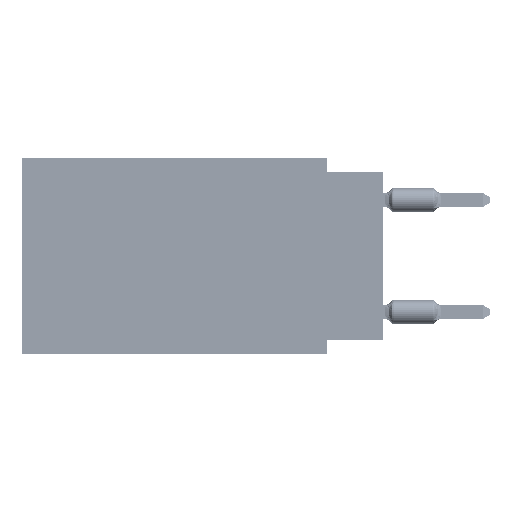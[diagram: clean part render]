
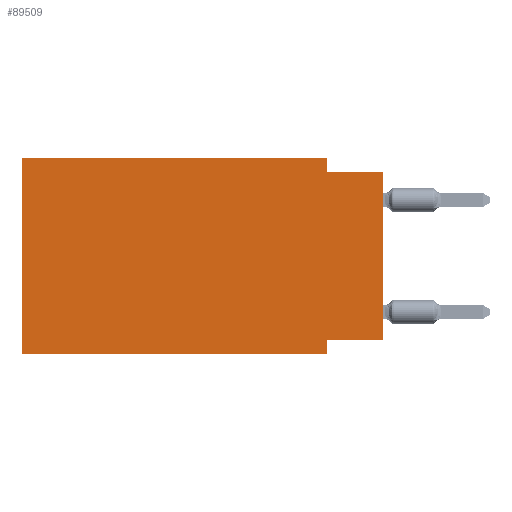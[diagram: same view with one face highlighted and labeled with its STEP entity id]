
A CAD part, left-side view. The second image highlights one B-rep face of the part: STEP entity #89509.
In plain terms, the highlighted planar face has unit normal (-1, 0, 0).
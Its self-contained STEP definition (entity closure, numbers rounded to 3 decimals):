
#2604 = DIRECTION ( 'NONE',  ( 0., 0., -1. ) ) ;
#7927 = EDGE_CURVE ( 'NONE', #21733, #20440, #15681, .T. ) ;
#8365 = CARTESIAN_POINT ( 'NONE',  ( 0., 16.383, -8.89 ) ) ;
#8653 = VECTOR ( 'NONE', #2604, 1000. ) ;
#8928 = DIRECTION ( 'NONE',  ( 0., -1., 0. ) ) ;
#9416 = CARTESIAN_POINT ( 'NONE',  ( 0., 16.383, 0. ) ) ;
#9968 = DIRECTION ( 'NONE',  ( 0., 0., -1. ) ) ;
#9999 = VECTOR ( 'NONE', #70797, 1000. ) ;
#10067 = DIRECTION ( 'NONE',  ( 0., 0., 1. ) ) ;
#15681 = LINE ( 'NONE', #32396, #109219 ) ;
#18236 = ORIENTED_EDGE ( 'NONE', *, *, #20844, .F. ) ;
#20440 = VERTEX_POINT ( 'NONE', #44941 ) ;
#20844 = EDGE_CURVE ( 'NONE', #87020, #33967, #105985, .T. ) ;
#21031 = CARTESIAN_POINT ( 'NONE',  ( 0., 2.54, 0. ) ) ;
#21733 = VERTEX_POINT ( 'NONE', #104017 ) ;
#23191 = CARTESIAN_POINT ( 'NONE',  ( 0., 2.54, -8.89 ) ) ;
#24398 = EDGE_CURVE ( 'NONE', #94822, #26685, #70625, .T. ) ;
#25597 = ORIENTED_EDGE ( 'NONE', *, *, #54971, .F. ) ;
#26632 = VECTOR ( 'NONE', #39932, 1000. ) ;
#26685 = VERTEX_POINT ( 'NONE', #106906 ) ;
#27922 = CARTESIAN_POINT ( 'NONE',  ( 0., 0., 0. ) ) ;
#28302 = VERTEX_POINT ( 'NONE', #31006 ) ;
#30061 = CARTESIAN_POINT ( 'NONE',  ( 0., 16.383, 0. ) ) ;
#30496 = VERTEX_POINT ( 'NONE', #94776 ) ;
#31006 = CARTESIAN_POINT ( 'NONE',  ( 0., 2.54, -0.635 ) ) ;
#32396 = CARTESIAN_POINT ( 'NONE',  ( 0., 16.383, 0. ) ) ;
#33326 = VECTOR ( 'NONE', #39279, 1000. ) ;
#33967 = VERTEX_POINT ( 'NONE', #63961 ) ;
#35767 = DIRECTION ( 'NONE',  ( 0., -1., 0. ) ) ;
#38302 = ORIENTED_EDGE ( 'NONE', *, *, #90954, .T. ) ;
#39279 = DIRECTION ( 'NONE',  ( 0., 0., 1. ) ) ;
#39932 = DIRECTION ( 'NONE',  ( 0., 0., -1. ) ) ;
#40236 = EDGE_CURVE ( 'NONE', #33967, #26685, #84927, .T. ) ;
#44941 = CARTESIAN_POINT ( 'NONE',  ( 0., 2.54, 0. ) ) ;
#46829 = FACE_OUTER_BOUND ( 'NONE', #102808, .T. ) ;
#54971 = EDGE_CURVE ( 'NONE', #20440, #28302, #64884, .T. ) ;
#60241 = ORIENTED_EDGE ( 'NONE', *, *, #78109, .F. ) ;
#63961 = CARTESIAN_POINT ( 'NONE',  ( 0., 2.54, -8.255 ) ) ;
#64884 = LINE ( 'NONE', #21031, #8653 ) ;
#66978 = LINE ( 'NONE', #30061, #33326 ) ;
#67086 = CARTESIAN_POINT ( 'NONE',  ( 0., 16.383, -8.89 ) ) ;
#70423 = LINE ( 'NONE', #80770, #74649 ) ;
#70625 = LINE ( 'NONE', #8365, #82214 ) ;
#70797 = DIRECTION ( 'NONE',  ( 0., 1., 0. ) ) ;
#71643 = CARTESIAN_POINT ( 'NONE',  ( 0., 0., -8.255 ) ) ;
#74649 = VECTOR ( 'NONE', #35767, 1000. ) ;
#78040 = ORIENTED_EDGE ( 'NONE', *, *, #24398, .T. ) ;
#78109 = EDGE_CURVE ( 'NONE', #28302, #30496, #70423, .T. ) ;
#79460 = CARTESIAN_POINT ( 'NONE',  ( 0., 0., -8.255 ) ) ;
#79778 = DIRECTION ( 'NONE',  ( 1., 0., 0. ) ) ;
#80770 = CARTESIAN_POINT ( 'NONE',  ( 0., 0., -0.635 ) ) ;
#82214 = VECTOR ( 'NONE', #8928, 1000. ) ;
#84927 = LINE ( 'NONE', #23191, #26632 ) ;
#86586 = ORIENTED_EDGE ( 'NONE', *, *, #7927, .F. ) ;
#87020 = VERTEX_POINT ( 'NONE', #71643 ) ;
#89509 = ADVANCED_FACE ( 'NONE', ( #46829 ), #106860, .F. ) ;
#90954 = EDGE_CURVE ( 'NONE', #87020, #30496, #98884, .T. ) ;
#91482 = EDGE_CURVE ( 'NONE', #94822, #21733, #66978, .T. ) ;
#94776 = CARTESIAN_POINT ( 'NONE',  ( 0., 0., -0.635 ) ) ;
#94822 = VERTEX_POINT ( 'NONE', #67086 ) ;
#97185 = ORIENTED_EDGE ( 'NONE', *, *, #40236, .F. ) ;
#98884 = LINE ( 'NONE', #27922, #101246 ) ;
#101246 = VECTOR ( 'NONE', #10067, 1000. ) ;
#101651 = DIRECTION ( 'NONE',  ( 0., -1., 0. ) ) ;
#102808 = EDGE_LOOP ( 'NONE', ( #38302, #60241, #25597, #86586, #106050, #78040, #97185, #18236 ) ) ;
#104017 = CARTESIAN_POINT ( 'NONE',  ( 0., 16.383, 0. ) ) ;
#105985 = LINE ( 'NONE', #79460, #9999 ) ;
#106050 = ORIENTED_EDGE ( 'NONE', *, *, #91482, .F. ) ;
#106753 = AXIS2_PLACEMENT_3D ( 'NONE', #9416, #79778, #9968 ) ;
#106860 = PLANE ( 'NONE',  #106753 ) ;
#106906 = CARTESIAN_POINT ( 'NONE',  ( 0., 2.54, -8.89 ) ) ;
#109219 = VECTOR ( 'NONE', #101651, 1000. ) ;
